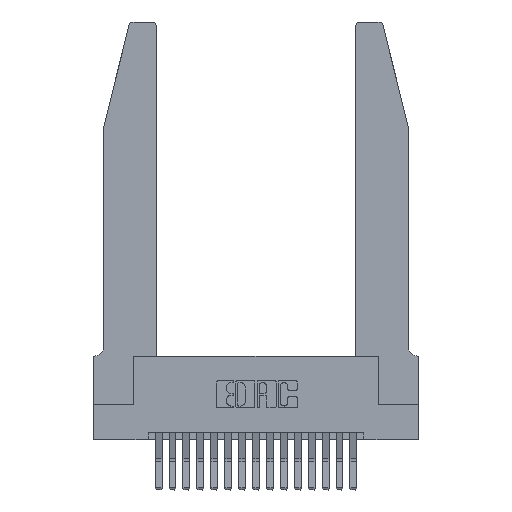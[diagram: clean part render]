
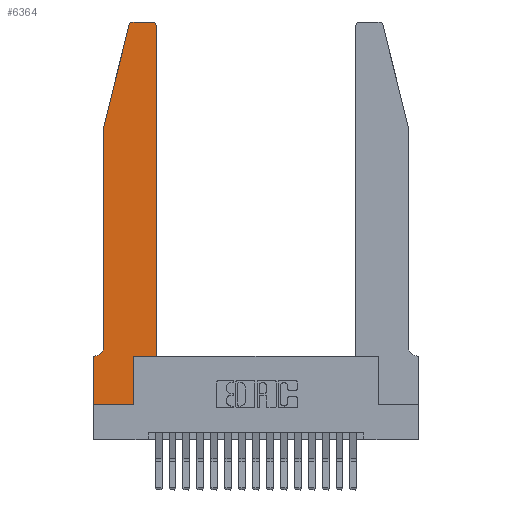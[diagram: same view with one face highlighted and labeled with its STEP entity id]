
A CAD part, top view. The second image highlights one B-rep face of the part: STEP entity #6364.
In plain terms, the highlighted planar face has unit normal (0, 0, 1).
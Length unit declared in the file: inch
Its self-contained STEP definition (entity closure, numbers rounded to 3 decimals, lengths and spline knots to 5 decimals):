
#192 = VERTEX_POINT ( 'NONE', #2817 ) ;
#220 = EDGE_CURVE ( 'NONE', #4137, #12742, #12344, .T. ) ;
#636 = VERTEX_POINT ( 'NONE', #17485 ) ;
#661 = LINE ( 'NONE', #12571, #12715 ) ;
#745 = DIRECTION ( 'NONE',  ( 1., 0., 0. ) ) ;
#807 = DIRECTION ( 'NONE',  ( 0., 0., 1. ) ) ;
#1227 = VECTOR ( 'NONE', #10900, 39.37008 ) ;
#1332 = LINE ( 'NONE', #19417, #9179 ) ;
#1749 = LINE ( 'NONE', #20162, #1227 ) ;
#1935 = CARTESIAN_POINT ( 'NONE',  ( 0., 0., 0.37 ) ) ;
#2457 = PLANE ( 'NONE',  #13775 ) ;
#2561 = LINE ( 'NONE', #2879, #14468 ) ;
#2817 = CARTESIAN_POINT ( 'NONE',  ( 0.0755, 0.42, 0.37 ) ) ;
#2879 = CARTESIAN_POINT ( 'NONE',  ( 0.4505, 0.35, 0.37 ) ) ;
#3033 = VERTEX_POINT ( 'NONE', #12767 ) ;
#4042 = AXIS2_PLACEMENT_3D ( 'NONE', #7841, #18655, #9380 ) ;
#4066 = CARTESIAN_POINT ( 'NONE',  ( 0., 0.35, 0.37 ) ) ;
#4092 = LINE ( 'NONE', #11182, #20062 ) ;
#4137 = VERTEX_POINT ( 'NONE', #13801 ) ;
#4150 = EDGE_LOOP ( 'NONE', ( #16804, #9067, #13204, #17305, #13682, #17781, #18261, #6422, #11009, #7392, #15624, #19711 ) ) ;
#4529 = VECTOR ( 'NONE', #17618, 39.37008 ) ;
#4689 = VERTEX_POINT ( 'NONE', #10712 ) ;
#4715 = CARTESIAN_POINT ( 'NONE',  ( 0., 0., 0.37 ) ) ;
#4827 = VERTEX_POINT ( 'NONE', #20087 ) ;
#4876 = CARTESIAN_POINT ( 'NONE',  ( 0.25487, 2.72718, 0.37 ) ) ;
#6364 = ADVANCED_FACE ( 'NONE', ( #13360 ), #2457, .T. ) ;
#6422 = ORIENTED_EDGE ( 'NONE', *, *, #9643, .T. ) ;
#6633 = EDGE_CURVE ( 'NONE', #192, #4689, #16721, .T. ) ;
#7141 = VECTOR ( 'NONE', #18002, 39.37008 ) ;
#7193 = CARTESIAN_POINT ( 'NONE',  ( 0.4505, 0.35, 0.37 ) ) ;
#7392 = ORIENTED_EDGE ( 'NONE', *, *, #20257, .T. ) ;
#7841 = CARTESIAN_POINT ( 'NONE',  ( 0.0055, 0.42, 0.37 ) ) ;
#8451 = EDGE_CURVE ( 'NONE', #3033, #4137, #2561, .T. ) ;
#8453 = CARTESIAN_POINT ( 'NONE',  ( 0., 0.35, 0.37 ) ) ;
#8743 = DIRECTION ( 'NONE',  ( 0., 0., 1. ) ) ;
#8873 = CARTESIAN_POINT ( 'NONE',  ( 0.4205, 2.75, 0.37 ) ) ;
#9067 = ORIENTED_EDGE ( 'NONE', *, *, #20234, .T. ) ;
#9179 = VECTOR ( 'NONE', #17872, 39.37008 ) ;
#9380 = DIRECTION ( 'NONE',  ( -1., 0., 0. ) ) ;
#9643 = EDGE_CURVE ( 'NONE', #15287, #4827, #1749, .T. ) ;
#9928 = CARTESIAN_POINT ( 'NONE',  ( 0.4205, 2.72, 0.37 ) ) ;
#9940 = DIRECTION ( 'NONE',  ( -1., 0., 0. ) ) ;
#10219 = CARTESIAN_POINT ( 'NONE',  ( 0.284, 2.72, 0.37 ) ) ;
#10401 = EDGE_CURVE ( 'NONE', #15174, #14059, #4092, .T. ) ;
#10673 = DIRECTION ( 'NONE',  ( 0., 1., 0. ) ) ;
#10712 = CARTESIAN_POINT ( 'NONE',  ( 0.0055, 0.35, 0.37 ) ) ;
#10900 = DIRECTION ( 'NONE',  ( 1., 0., 0. ) ) ;
#11009 = ORIENTED_EDGE ( 'NONE', *, *, #16879, .T. ) ;
#11055 = DIRECTION ( 'NONE',  ( 0., -1., 0. ) ) ;
#11182 = CARTESIAN_POINT ( 'NONE',  ( 0.0755, 2., 0.37 ) ) ;
#11258 = VERTEX_POINT ( 'NONE', #8453 ) ;
#11290 = VERTEX_POINT ( 'NONE', #19253 ) ;
#11695 = AXIS2_PLACEMENT_3D ( 'NONE', #10219, #807, #11811 ) ;
#11811 = DIRECTION ( 'NONE',  ( 1., 0., 0. ) ) ;
#11887 = EDGE_CURVE ( 'NONE', #12742, #636, #15917, .T. ) ;
#12156 = VECTOR ( 'NONE', #17083, 39.37008 ) ;
#12219 = DIRECTION ( 'NONE',  ( 0., 0., 1. ) ) ;
#12344 = CIRCLE ( 'NONE', #16664, 0.03 ) ;
#12571 = CARTESIAN_POINT ( 'NONE',  ( 0.0755, 2., 0.37 ) ) ;
#12715 = VECTOR ( 'NONE', #11055, 39.37008 ) ;
#12742 = VERTEX_POINT ( 'NONE', #8873 ) ;
#12759 = DIRECTION ( 'NONE',  ( -0.239, -0.971, 0. ) ) ;
#12767 = CARTESIAN_POINT ( 'NONE',  ( 0.4505, 0.35, 0.37 ) ) ;
#13204 = ORIENTED_EDGE ( 'NONE', *, *, #10401, .T. ) ;
#13360 = FACE_OUTER_BOUND ( 'NONE', #4150, .T. ) ;
#13682 = ORIENTED_EDGE ( 'NONE', *, *, #6633, .T. ) ;
#13775 = AXIS2_PLACEMENT_3D ( 'NONE', #4066, #8743, #19547 ) ;
#13801 = CARTESIAN_POINT ( 'NONE',  ( 0.4505, 2.72, 0.37 ) ) ;
#13943 = EDGE_CURVE ( 'NONE', #14059, #192, #661, .T. ) ;
#14059 = VERTEX_POINT ( 'NONE', #17478 ) ;
#14468 = VECTOR ( 'NONE', #10673, 39.37008 ) ;
#14511 = CARTESIAN_POINT ( 'NONE',  ( 0.2605, 2.75, 0.37 ) ) ;
#15174 = VERTEX_POINT ( 'NONE', #4876 ) ;
#15287 = VERTEX_POINT ( 'NONE', #1935 ) ;
#15363 = CIRCLE ( 'NONE', #11695, 0.03 ) ;
#15624 = ORIENTED_EDGE ( 'NONE', *, *, #8451, .T. ) ;
#15725 = EDGE_CURVE ( 'NONE', #11258, #15287, #16258, .T. ) ;
#15917 = LINE ( 'NONE', #14511, #4529 ) ;
#16258 = LINE ( 'NONE', #4715, #12156 ) ;
#16664 = AXIS2_PLACEMENT_3D ( 'NONE', #9928, #12219, #745 ) ;
#16721 = CIRCLE ( 'NONE', #4042, 0.07 ) ;
#16763 = EDGE_CURVE ( 'NONE', #4689, #11258, #19342, .T. ) ;
#16804 = ORIENTED_EDGE ( 'NONE', *, *, #11887, .T. ) ;
#16879 = EDGE_CURVE ( 'NONE', #4827, #11290, #1332, .T. ) ;
#17083 = DIRECTION ( 'NONE',  ( 0., -1., 0. ) ) ;
#17305 = ORIENTED_EDGE ( 'NONE', *, *, #13943, .T. ) ;
#17478 = CARTESIAN_POINT ( 'NONE',  ( 0.0755, 2., 0.37 ) ) ;
#17485 = CARTESIAN_POINT ( 'NONE',  ( 0.284, 2.75, 0.37 ) ) ;
#17618 = DIRECTION ( 'NONE',  ( -1., 0., 0. ) ) ;
#17781 = ORIENTED_EDGE ( 'NONE', *, *, #16763, .T. ) ;
#17872 = DIRECTION ( 'NONE',  ( 0., 1., 0. ) ) ;
#18002 = DIRECTION ( 'NONE',  ( 1., 0., 0. ) ) ;
#18261 = ORIENTED_EDGE ( 'NONE', *, *, #15725, .T. ) ;
#18655 = DIRECTION ( 'NONE',  ( 0., 0., -1. ) ) ;
#18984 = LINE ( 'NONE', #7193, #7141 ) ;
#19211 = CARTESIAN_POINT ( 'NONE',  ( 0.0755, 0.35, 0.37 ) ) ;
#19253 = CARTESIAN_POINT ( 'NONE',  ( 0.2865, 0.35, 0.37 ) ) ;
#19342 = LINE ( 'NONE', #19211, #19824 ) ;
#19417 = CARTESIAN_POINT ( 'NONE',  ( 0.2865, 0.35, 0.37 ) ) ;
#19547 = DIRECTION ( 'NONE',  ( 1., 0., 0. ) ) ;
#19711 = ORIENTED_EDGE ( 'NONE', *, *, #220, .T. ) ;
#19824 = VECTOR ( 'NONE', #9940, 39.37008 ) ;
#20062 = VECTOR ( 'NONE', #12759, 39.37008 ) ;
#20087 = CARTESIAN_POINT ( 'NONE',  ( 0.2865, 0., 0.37 ) ) ;
#20162 = CARTESIAN_POINT ( 'NONE',  ( 0., 0., 0.37 ) ) ;
#20234 = EDGE_CURVE ( 'NONE', #636, #15174, #15363, .T. ) ;
#20257 = EDGE_CURVE ( 'NONE', #11290, #3033, #18984, .T. ) ;
